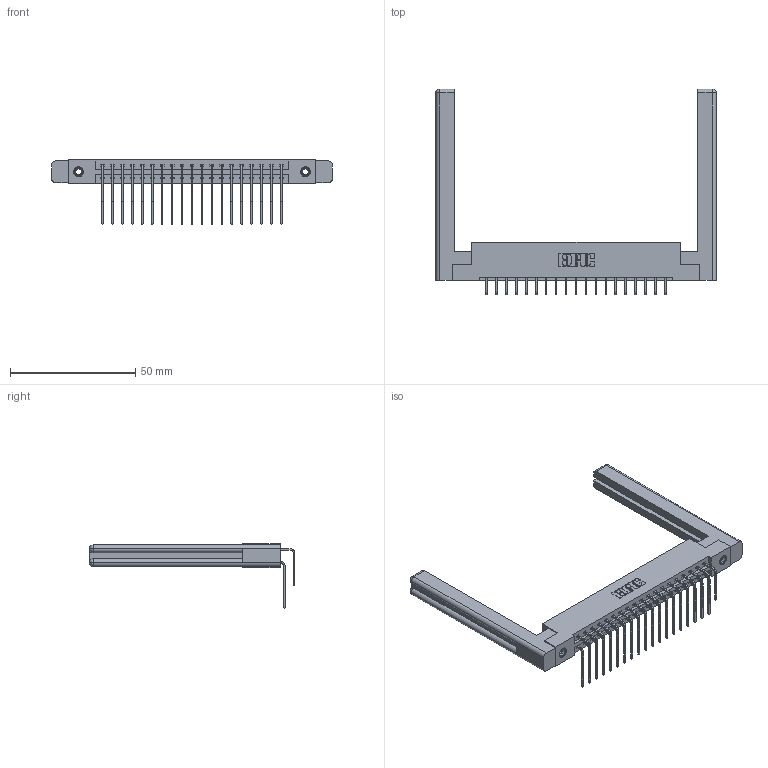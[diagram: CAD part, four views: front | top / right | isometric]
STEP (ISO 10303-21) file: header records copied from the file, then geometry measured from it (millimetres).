
FILE_DESCRIPTION (( 'STEP AP203' ), '1' );
FILE_NAME ('387-038-559-258.STEP', '2019-10-17T22:35:21', ( '' ), ( '' ), 'SwSTEP 2.0', 'SolidWorks 2016', '' );
FILE_SCHEMA (( 'CONFIG_CONTROL_DESIGN' ));
Length unit declared in the file: inch
Products named in the file (6): 345-292-001_558 559 Tail - 1; 307-220-058; 387-038-559-258; 345-250-001_345-250-001-102; 337 Part_Flush Mounting Lugs - 0.156 Dia-TI; 345-292-001_559 Tail - 2
Assembly tree (43 placements, depth 2):
  387-038-559-258
    337 Part_Flush Mounting Lugs - 0.156 Dia-TI
    345-292-001_558 559 Tail - 1  x19
    345-292-001_559 Tail - 2  x19
    345-250-001_345-250-001-102  x2
    307-220-058  x2
Bounding box: 111.91 x 81.98 x 25.53 mm (x, y, z)
Volume: 18849.6 mm3; surface area: 19159.1 mm2
Topology: 43 solids, 43 shells, 2384 faces, 7011 edges, 4610 vertices
Faces by surface type: plane 1674, cylinder 686, cone 12, torus 12
Entity records: 22124 total; most frequent: CARTESIAN_POINT 3800, ORIENTED_EDGE 3624, DIRECTION 3272, EDGE_CURVE 1812, VECTOR 1596, LINE 1596, VERTEX_POINT 1198, AXIS2_PLACEMENT_3D 838
